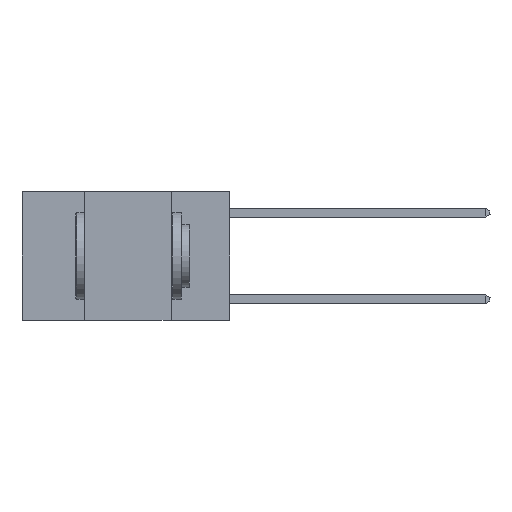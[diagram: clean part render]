
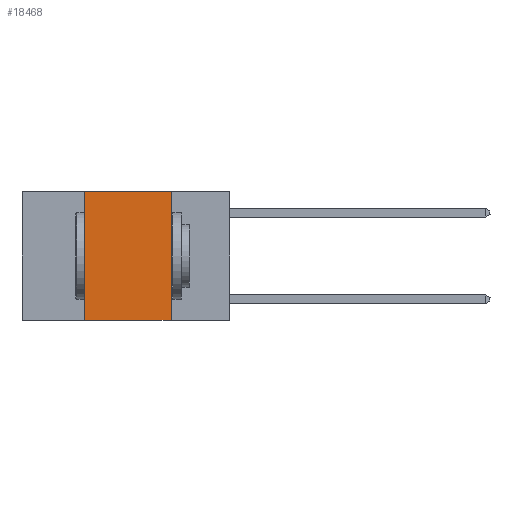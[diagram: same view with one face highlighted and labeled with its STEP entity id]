
A CAD part, left-side view. The second image highlights one B-rep face of the part: STEP entity #18468.
In plain terms, the highlighted planar face has unit normal (-1, 0, 0).
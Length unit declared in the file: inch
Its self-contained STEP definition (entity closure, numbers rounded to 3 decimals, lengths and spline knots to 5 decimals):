
#277 = CARTESIAN_POINT ( 'NONE',  ( 0., 0.6, 0. ) ) ;
#722 = CARTESIAN_POINT ( 'NONE',  ( 0., 0.42, 0. ) ) ;
#1118 = CARTESIAN_POINT ( 'NONE',  ( 0., 0.6, 0. ) ) ;
#1268 = ORIENTED_EDGE ( 'NONE', *, *, #2368, .F. ) ;
#2310 = DIRECTION ( 'NONE',  ( 0., 0., 1. ) ) ;
#2368 = EDGE_CURVE ( 'NONE', #24185, #13800, #18000, .T. ) ;
#4810 = EDGE_CURVE ( 'NONE', #8710, #21082, #20832, .T. ) ;
#6677 = LINE ( 'NONE', #1118, #16524 ) ;
#8710 = VERTEX_POINT ( 'NONE', #24845 ) ;
#9121 = DIRECTION ( 'NONE',  ( 0., 0., -1. ) ) ;
#11057 = ORIENTED_EDGE ( 'NONE', *, *, #4810, .F. ) ;
#11519 = VECTOR ( 'NONE', #9121, 39.37008 ) ;
#11562 = PLANE ( 'NONE',  #22589 ) ;
#12075 = EDGE_CURVE ( 'NONE', #8710, #13800, #25785, .T. ) ;
#13032 = DIRECTION ( 'NONE',  ( 0., -1., 0. ) ) ;
#13587 = DIRECTION ( 'NONE',  ( 0., -1., 0. ) ) ;
#13800 = VERTEX_POINT ( 'NONE', #16825 ) ;
#14314 = ORIENTED_EDGE ( 'NONE', *, *, #12075, .T. ) ;
#15215 = VECTOR ( 'NONE', #2310, 39.37008 ) ;
#16342 = ORIENTED_EDGE ( 'NONE', *, *, #18342, .F. ) ;
#16524 = VECTOR ( 'NONE', #13032, 39.37008 ) ;
#16825 = CARTESIAN_POINT ( 'NONE',  ( 0., 0.17, -0.37 ) ) ;
#18000 = LINE ( 'NONE', #21392, #11519 ) ;
#18342 = EDGE_CURVE ( 'NONE', #21082, #24185, #6677, .T. ) ;
#18468 = ADVANCED_FACE ( 'NONE', ( #21762 ), #11562, .F. ) ;
#18506 = DIRECTION ( 'NONE',  ( 1., 0., 0. ) ) ;
#19655 = CARTESIAN_POINT ( 'NONE',  ( 0., 0.6, -0.37 ) ) ;
#20812 = CARTESIAN_POINT ( 'NONE',  ( 0., 0.42, 0. ) ) ;
#20832 = LINE ( 'NONE', #722, #15215 ) ;
#20923 = DIRECTION ( 'NONE',  ( 0., 0., -1. ) ) ;
#21082 = VERTEX_POINT ( 'NONE', #20812 ) ;
#21392 = CARTESIAN_POINT ( 'NONE',  ( 0., 0.17, 0. ) ) ;
#21762 = FACE_OUTER_BOUND ( 'NONE', #25175, .T. ) ;
#22589 = AXIS2_PLACEMENT_3D ( 'NONE', #277, #18506, #20923 ) ;
#23787 = CARTESIAN_POINT ( 'NONE',  ( 0., 0.17, 0. ) ) ;
#24185 = VERTEX_POINT ( 'NONE', #23787 ) ;
#24845 = CARTESIAN_POINT ( 'NONE',  ( 0., 0.42, -0.37 ) ) ;
#25175 = EDGE_LOOP ( 'NONE', ( #1268, #16342, #11057, #14314 ) ) ;
#25785 = LINE ( 'NONE', #19655, #25843 ) ;
#25843 = VECTOR ( 'NONE', #13587, 39.37008 ) ;
